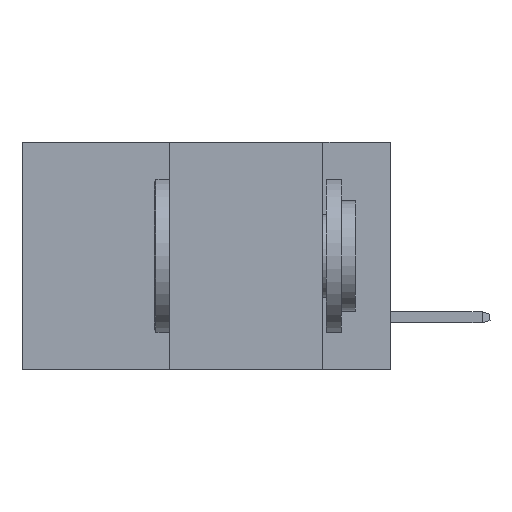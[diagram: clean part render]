
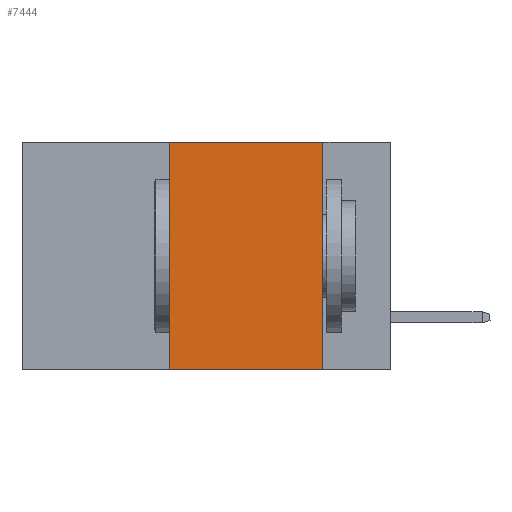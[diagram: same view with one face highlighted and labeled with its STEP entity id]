
A CAD part, left-side view. The second image highlights one B-rep face of the part: STEP entity #7444.
In plain terms, the highlighted planar face has unit normal (-1, 0, 0).
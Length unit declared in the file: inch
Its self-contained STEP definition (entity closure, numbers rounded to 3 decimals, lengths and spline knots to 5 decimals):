
#415 = LINE ( 'NONE', #4020, #18952 ) ;
#586 = EDGE_CURVE ( 'NONE', #8738, #13684, #22161, .T. ) ;
#816 = VERTEX_POINT ( 'NONE', #22469 ) ;
#2330 = AXIS2_PLACEMENT_3D ( 'NONE', #16165, #7396, #19741 ) ;
#3732 = PLANE ( 'NONE',  #2330 ) ;
#4020 = CARTESIAN_POINT ( 'NONE',  ( 0., 0.36, 0. ) ) ;
#5186 = DIRECTION ( 'NONE',  ( 0., 0., -1. ) ) ;
#5570 = VECTOR ( 'NONE', #5186, 39.37008 ) ;
#5766 = ORIENTED_EDGE ( 'NONE', *, *, #13581, .F. ) ;
#6006 = ORIENTED_EDGE ( 'NONE', *, *, #586, .F. ) ;
#6064 = ORIENTED_EDGE ( 'NONE', *, *, #11262, .F. ) ;
#6068 = ORIENTED_EDGE ( 'NONE', *, *, #6488, .T. ) ;
#6488 = EDGE_CURVE ( 'NONE', #10530, #816, #13786, .T. ) ;
#7396 = DIRECTION ( 'NONE',  ( 1., 0., 0. ) ) ;
#7444 = ADVANCED_FACE ( 'NONE', ( #22344 ), #3732, .F. ) ;
#8119 = VECTOR ( 'NONE', #14287, 39.37008 ) ;
#8738 = VERTEX_POINT ( 'NONE', #8814 ) ;
#8814 = CARTESIAN_POINT ( 'NONE',  ( 0., 0.36, 0. ) ) ;
#9494 = DIRECTION ( 'NONE',  ( 0., 0., 1. ) ) ;
#10530 = VERTEX_POINT ( 'NONE', #13919 ) ;
#11262 = EDGE_CURVE ( 'NONE', #10530, #8738, #415, .T. ) ;
#11466 = DIRECTION ( 'NONE',  ( 0., -1., 0. ) ) ;
#12699 = CARTESIAN_POINT ( 'NONE',  ( 0., 0.6, 0. ) ) ;
#13266 = VECTOR ( 'NONE', #11466, 39.37008 ) ;
#13581 = EDGE_CURVE ( 'NONE', #13684, #816, #15012, .T. ) ;
#13684 = VERTEX_POINT ( 'NONE', #21442 ) ;
#13786 = LINE ( 'NONE', #16770, #13266 ) ;
#13919 = CARTESIAN_POINT ( 'NONE',  ( 0., 0.36, -0.37 ) ) ;
#14287 = DIRECTION ( 'NONE',  ( 0., -1., 0. ) ) ;
#15012 = LINE ( 'NONE', #17594, #5570 ) ;
#16165 = CARTESIAN_POINT ( 'NONE',  ( 0., 0.6, 0. ) ) ;
#16770 = CARTESIAN_POINT ( 'NONE',  ( 0., 0.6, -0.37 ) ) ;
#17594 = CARTESIAN_POINT ( 'NONE',  ( 0., 0.11, 0. ) ) ;
#18952 = VECTOR ( 'NONE', #9494, 39.37008 ) ;
#19741 = DIRECTION ( 'NONE',  ( 0., 0., -1. ) ) ;
#21442 = CARTESIAN_POINT ( 'NONE',  ( 0., 0.11, 0. ) ) ;
#22161 = LINE ( 'NONE', #12699, #8119 ) ;
#22344 = FACE_OUTER_BOUND ( 'NONE', #22964, .T. ) ;
#22469 = CARTESIAN_POINT ( 'NONE',  ( 0., 0.11, -0.37 ) ) ;
#22964 = EDGE_LOOP ( 'NONE', ( #5766, #6006, #6064, #6068 ) ) ;
